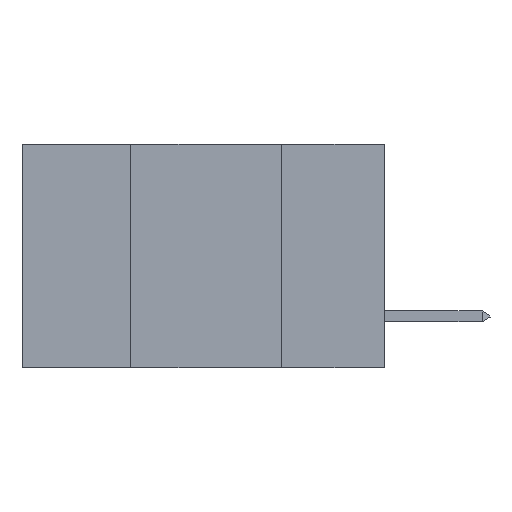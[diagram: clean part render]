
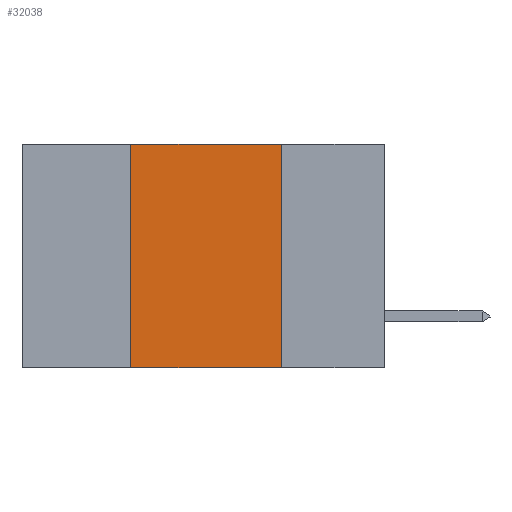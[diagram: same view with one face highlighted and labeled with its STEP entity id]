
A CAD part, left-side view. The second image highlights one B-rep face of the part: STEP entity #32038.
In plain terms, the highlighted planar face has unit normal (-1, 0, 0).
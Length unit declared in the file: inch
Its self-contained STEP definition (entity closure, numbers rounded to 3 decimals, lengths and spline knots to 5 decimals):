
#391 = DIRECTION ( 'NONE',  ( 1., 0., 0. ) ) ;
#612 = VECTOR ( 'NONE', #25410, 39.37008 ) ;
#645 = ORIENTED_EDGE ( 'NONE', *, *, #33860, .T. ) ;
#2582 = LINE ( 'NONE', #19740, #5530 ) ;
#4446 = VERTEX_POINT ( 'NONE', #34885 ) ;
#5530 = VECTOR ( 'NONE', #17301, 39.37008 ) ;
#5942 = EDGE_LOOP ( 'NONE', ( #11905, #11529, #25618, #645 ) ) ;
#7407 = AXIS2_PLACEMENT_3D ( 'NONE', #33802, #391, #19900 ) ;
#8300 = CARTESIAN_POINT ( 'NONE',  ( 0., 0.6, -0.37 ) ) ;
#11112 = LINE ( 'NONE', #34133, #25233 ) ;
#11529 = ORIENTED_EDGE ( 'NONE', *, *, #12051, .F. ) ;
#11905 = ORIENTED_EDGE ( 'NONE', *, *, #24398, .F. ) ;
#12051 = EDGE_CURVE ( 'NONE', #23130, #17825, #11112, .T. ) ;
#14278 = PLANE ( 'NONE',  #7407 ) ;
#15377 = VERTEX_POINT ( 'NONE', #22336 ) ;
#17301 = DIRECTION ( 'NONE',  ( 0., 0., -1. ) ) ;
#17425 = DIRECTION ( 'NONE',  ( 0., -1., 0. ) ) ;
#17825 = VERTEX_POINT ( 'NONE', #20593 ) ;
#19461 = CARTESIAN_POINT ( 'NONE',  ( 0., 0.42, 0. ) ) ;
#19580 = LINE ( 'NONE', #28487, #30911 ) ;
#19740 = CARTESIAN_POINT ( 'NONE',  ( 0., 0.17, 0. ) ) ;
#19900 = DIRECTION ( 'NONE',  ( 0., 0., -1. ) ) ;
#20593 = CARTESIAN_POINT ( 'NONE',  ( 0., 0.17, 0. ) ) ;
#22336 = CARTESIAN_POINT ( 'NONE',  ( 0., 0.42, -0.37 ) ) ;
#23130 = VERTEX_POINT ( 'NONE', #19461 ) ;
#24398 = EDGE_CURVE ( 'NONE', #17825, #4446, #2582, .T. ) ;
#25233 = VECTOR ( 'NONE', #17425, 39.37008 ) ;
#25410 = DIRECTION ( 'NONE',  ( 0., -1., 0. ) ) ;
#25618 = ORIENTED_EDGE ( 'NONE', *, *, #29587, .F. ) ;
#25778 = DIRECTION ( 'NONE',  ( 0., 0., 1. ) ) ;
#28487 = CARTESIAN_POINT ( 'NONE',  ( 0., 0.42, 0. ) ) ;
#29587 = EDGE_CURVE ( 'NONE', #15377, #23130, #19580, .T. ) ;
#30911 = VECTOR ( 'NONE', #25778, 39.37008 ) ;
#31147 = LINE ( 'NONE', #8300, #612 ) ;
#31717 = FACE_OUTER_BOUND ( 'NONE', #5942, .T. ) ;
#32038 = ADVANCED_FACE ( 'NONE', ( #31717 ), #14278, .F. ) ;
#33802 = CARTESIAN_POINT ( 'NONE',  ( 0., 0.6, 0. ) ) ;
#33860 = EDGE_CURVE ( 'NONE', #15377, #4446, #31147, .T. ) ;
#34133 = CARTESIAN_POINT ( 'NONE',  ( 0., 0.6, 0. ) ) ;
#34885 = CARTESIAN_POINT ( 'NONE',  ( 0., 0.17, -0.37 ) ) ;
